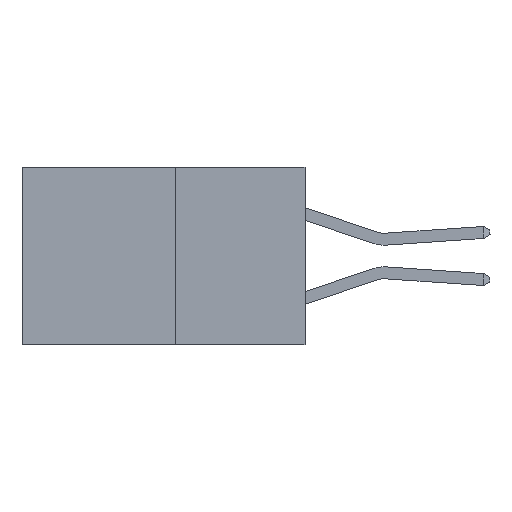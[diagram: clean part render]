
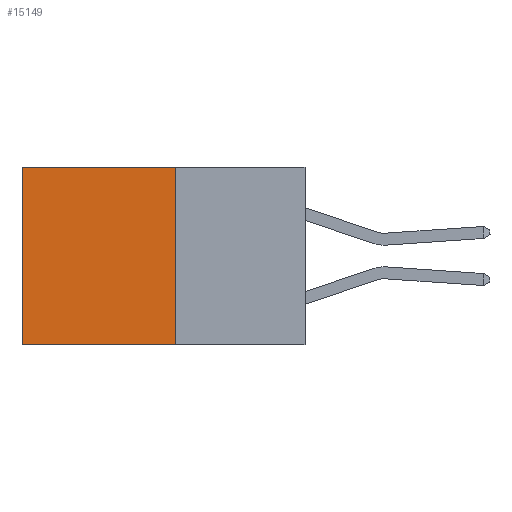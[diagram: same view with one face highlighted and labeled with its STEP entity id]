
A CAD part, left-side view. The second image highlights one B-rep face of the part: STEP entity #15149.
In plain terms, the highlighted planar face has unit normal (-1, 0, 0).
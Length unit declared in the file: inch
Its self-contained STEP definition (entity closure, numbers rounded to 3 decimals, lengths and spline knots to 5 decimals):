
#30 = VECTOR ( 'NONE', #6595, 39.37008 ) ;
#947 = VERTEX_POINT ( 'NONE', #8167 ) ;
#1005 = LINE ( 'NONE', #1131, #15171 ) ;
#1131 = CARTESIAN_POINT ( 'NONE',  ( 0.277, 0.27, -0.37 ) ) ;
#1245 = ORIENTED_EDGE ( 'NONE', *, *, #15758, .F. ) ;
#1444 = VERTEX_POINT ( 'NONE', #12985 ) ;
#1754 = ORIENTED_EDGE ( 'NONE', *, *, #6111, .T. ) ;
#2271 = ORIENTED_EDGE ( 'NONE', *, *, #6890, .T. ) ;
#3004 = VECTOR ( 'NONE', #10076, 39.37008 ) ;
#3524 = EDGE_CURVE ( 'NONE', #11261, #1444, #14156, .T. ) ;
#3942 = ORIENTED_EDGE ( 'NONE', *, *, #3524, .F. ) ;
#3986 = CARTESIAN_POINT ( 'NONE',  ( 0.277, 0.27, 0. ) ) ;
#4033 = CARTESIAN_POINT ( 'NONE',  ( 0.277, 0.27, -0.37 ) ) ;
#6109 = EDGE_LOOP ( 'NONE', ( #2271, #1245, #3942, #1754 ) ) ;
#6111 = EDGE_CURVE ( 'NONE', #11261, #947, #12999, .T. ) ;
#6230 = DIRECTION ( 'NONE',  ( 0., 0., -1. ) ) ;
#6258 = DIRECTION ( 'NONE',  ( 1., 0., 0. ) ) ;
#6595 = DIRECTION ( 'NONE',  ( 0., 0., -1. ) ) ;
#6626 = PLANE ( 'NONE',  #13393 ) ;
#6890 = EDGE_CURVE ( 'NONE', #947, #13611, #15122, .T. ) ;
#8167 = CARTESIAN_POINT ( 'NONE',  ( 0.277, 0.59, 0. ) ) ;
#8403 = DIRECTION ( 'NONE',  ( 0., 1., 0. ) ) ;
#8855 = CARTESIAN_POINT ( 'NONE',  ( 0.277, 0.59, -0.37 ) ) ;
#8912 = CARTESIAN_POINT ( 'NONE',  ( 0.277, 0.59, -0.37 ) ) ;
#10076 = DIRECTION ( 'NONE',  ( 0., 0., -1. ) ) ;
#10273 = VECTOR ( 'NONE', #16204, 39.37008 ) ;
#11261 = VERTEX_POINT ( 'NONE', #3986 ) ;
#11931 = CARTESIAN_POINT ( 'NONE',  ( 0.277, 0.27, -0.37 ) ) ;
#12985 = CARTESIAN_POINT ( 'NONE',  ( 0.277, 0.27, -0.37 ) ) ;
#12999 = LINE ( 'NONE', #17282, #10273 ) ;
#13393 = AXIS2_PLACEMENT_3D ( 'NONE', #4033, #6258, #6230 ) ;
#13611 = VERTEX_POINT ( 'NONE', #8912 ) ;
#14156 = LINE ( 'NONE', #11931, #3004 ) ;
#14554 = FACE_OUTER_BOUND ( 'NONE', #6109, .T. ) ;
#15122 = LINE ( 'NONE', #8855, #30 ) ;
#15149 = ADVANCED_FACE ( 'NONE', ( #14554 ), #6626, .F. ) ;
#15171 = VECTOR ( 'NONE', #8403, 39.37008 ) ;
#15758 = EDGE_CURVE ( 'NONE', #1444, #13611, #1005, .T. ) ;
#16204 = DIRECTION ( 'NONE',  ( 0., 1., 0. ) ) ;
#17282 = CARTESIAN_POINT ( 'NONE',  ( 0.277, 0.27, 0. ) ) ;
